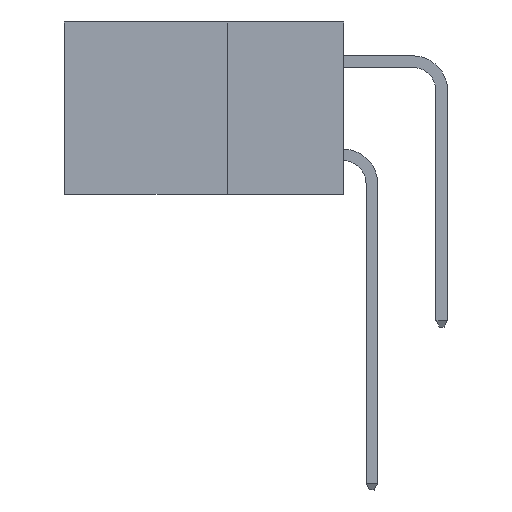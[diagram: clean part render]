
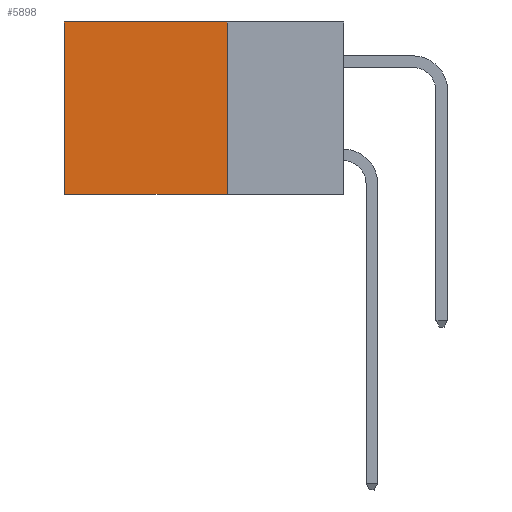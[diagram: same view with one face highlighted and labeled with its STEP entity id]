
A CAD part, left-side view. The second image highlights one B-rep face of the part: STEP entity #5898.
In plain terms, the highlighted planar face has unit normal (-1, 0, 0).
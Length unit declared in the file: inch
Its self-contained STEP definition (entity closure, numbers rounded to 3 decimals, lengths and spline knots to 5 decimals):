
#51 = ORIENTED_EDGE ( 'NONE', *, *, #18185, .T. ) ;
#331 = EDGE_CURVE ( 'NONE', #5390, #18613, #13970, .T. ) ;
#1099 = CARTESIAN_POINT ( 'NONE',  ( 0.298, 0.25, 0. ) ) ;
#3240 = LINE ( 'NONE', #23904, #14432 ) ;
#3404 = EDGE_CURVE ( 'NONE', #21632, #5390, #3240, .T. ) ;
#5390 = VERTEX_POINT ( 'NONE', #21635 ) ;
#5795 = FACE_OUTER_BOUND ( 'NONE', #24950, .T. ) ;
#5898 = ADVANCED_FACE ( 'NONE', ( #5795 ), #11475, .F. ) ;
#7557 = DIRECTION ( 'NONE',  ( 0., 1., 0. ) ) ;
#7707 = VECTOR ( 'NONE', #22318, 39.37008 ) ;
#8595 = DIRECTION ( 'NONE',  ( 0., 0., -1. ) ) ;
#9823 = VECTOR ( 'NONE', #8595, 39.37008 ) ;
#10527 = ORIENTED_EDGE ( 'NONE', *, *, #3404, .F. ) ;
#10723 = ORIENTED_EDGE ( 'NONE', *, *, #14748, .T. ) ;
#10790 = CARTESIAN_POINT ( 'NONE',  ( 0.298, 0.6, 0. ) ) ;
#10911 = CARTESIAN_POINT ( 'NONE',  ( 0.298, 0.6, -0.37 ) ) ;
#11475 = PLANE ( 'NONE',  #24995 ) ;
#11824 = VERTEX_POINT ( 'NONE', #10790 ) ;
#13208 = DIRECTION ( 'NONE',  ( 1., 0., 0. ) ) ;
#13487 = CARTESIAN_POINT ( 'NONE',  ( 0.298, 0.25, 0. ) ) ;
#13970 = LINE ( 'NONE', #18091, #7707 ) ;
#14432 = VECTOR ( 'NONE', #23732, 39.37008 ) ;
#14627 = CARTESIAN_POINT ( 'NONE',  ( 0.298, 0.6, 0. ) ) ;
#14748 = EDGE_CURVE ( 'NONE', #21632, #11824, #22682, .T. ) ;
#15223 = DIRECTION ( 'NONE',  ( 0., 0., -1. ) ) ;
#16376 = LINE ( 'NONE', #14627, #9823 ) ;
#18091 = CARTESIAN_POINT ( 'NONE',  ( 0.298, 0.25, -0.37 ) ) ;
#18185 = EDGE_CURVE ( 'NONE', #11824, #18613, #16376, .T. ) ;
#18613 = VERTEX_POINT ( 'NONE', #10911 ) ;
#20033 = ORIENTED_EDGE ( 'NONE', *, *, #331, .F. ) ;
#21632 = VERTEX_POINT ( 'NONE', #1099 ) ;
#21635 = CARTESIAN_POINT ( 'NONE',  ( 0.298, 0.25, -0.37 ) ) ;
#22318 = DIRECTION ( 'NONE',  ( 0., 1., 0. ) ) ;
#22682 = LINE ( 'NONE', #13487, #24249 ) ;
#23732 = DIRECTION ( 'NONE',  ( 0., 0., -1. ) ) ;
#23904 = CARTESIAN_POINT ( 'NONE',  ( 0.298, 0.25, 0. ) ) ;
#24249 = VECTOR ( 'NONE', #7557, 39.37008 ) ;
#24950 = EDGE_LOOP ( 'NONE', ( #51, #20033, #10527, #10723 ) ) ;
#24995 = AXIS2_PLACEMENT_3D ( 'NONE', #25471, #13208, #15223 ) ;
#25471 = CARTESIAN_POINT ( 'NONE',  ( 0.298, 0.25, 0. ) ) ;
